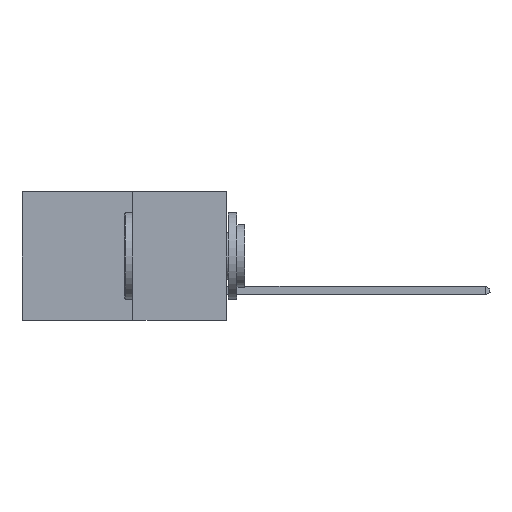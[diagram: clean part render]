
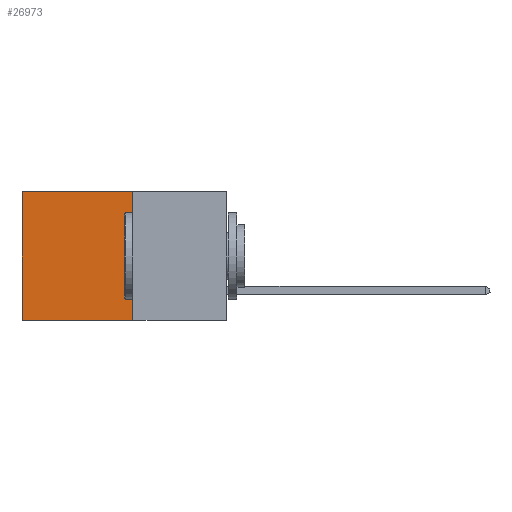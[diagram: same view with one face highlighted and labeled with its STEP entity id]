
A CAD part, left-side view. The second image highlights one B-rep face of the part: STEP entity #26973.
In plain terms, the highlighted planar face has unit normal (-1, 0, 0).
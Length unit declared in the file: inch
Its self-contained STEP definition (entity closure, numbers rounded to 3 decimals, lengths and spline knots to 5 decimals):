
#985 = LINE ( 'NONE', #19650, #26317 ) ;
#1512 = VERTEX_POINT ( 'NONE', #6569 ) ;
#2138 = VECTOR ( 'NONE', #2376, 39.37008 ) ;
#2376 = DIRECTION ( 'NONE',  ( 0., 1., 0. ) ) ;
#3024 = CARTESIAN_POINT ( 'NONE',  ( 0.277, 0.27, -0.37 ) ) ;
#3269 = VERTEX_POINT ( 'NONE', #3748 ) ;
#3719 = DIRECTION ( 'NONE',  ( 0., 1., 0. ) ) ;
#3748 = CARTESIAN_POINT ( 'NONE',  ( 0.277, 0.59, 0. ) ) ;
#5266 = LINE ( 'NONE', #24656, #11060 ) ;
#5448 = DIRECTION ( 'NONE',  ( 0., 0., -1. ) ) ;
#6569 = CARTESIAN_POINT ( 'NONE',  ( 0.277, 0.59, -0.37 ) ) ;
#6896 = LINE ( 'NONE', #23371, #25718 ) ;
#8676 = LINE ( 'NONE', #26833, #2138 ) ;
#9875 = AXIS2_PLACEMENT_3D ( 'NONE', #3024, #20206, #5448 ) ;
#10342 = VERTEX_POINT ( 'NONE', #30927 ) ;
#11060 = VECTOR ( 'NONE', #17388, 39.37008 ) ;
#11911 = EDGE_CURVE ( 'NONE', #22059, #10342, #5266, .T. ) ;
#12427 = ORIENTED_EDGE ( 'NONE', *, *, #29948, .F. ) ;
#14367 = EDGE_CURVE ( 'NONE', #3269, #1512, #985, .T. ) ;
#17032 = ORIENTED_EDGE ( 'NONE', *, *, #27685, .T. ) ;
#17388 = DIRECTION ( 'NONE',  ( 0., 0., -1. ) ) ;
#17759 = PLANE ( 'NONE',  #9875 ) ;
#19650 = CARTESIAN_POINT ( 'NONE',  ( 0.277, 0.59, -0.37 ) ) ;
#20057 = EDGE_LOOP ( 'NONE', ( #22193, #12427, #22409, #17032 ) ) ;
#20206 = DIRECTION ( 'NONE',  ( 1., 0., 0. ) ) ;
#21181 = FACE_OUTER_BOUND ( 'NONE', #20057, .T. ) ;
#22059 = VERTEX_POINT ( 'NONE', #22129 ) ;
#22129 = CARTESIAN_POINT ( 'NONE',  ( 0.277, 0.27, 0. ) ) ;
#22193 = ORIENTED_EDGE ( 'NONE', *, *, #14367, .T. ) ;
#22409 = ORIENTED_EDGE ( 'NONE', *, *, #11911, .F. ) ;
#23371 = CARTESIAN_POINT ( 'NONE',  ( 0.277, 0.27, 0. ) ) ;
#24656 = CARTESIAN_POINT ( 'NONE',  ( 0.277, 0.27, -0.37 ) ) ;
#25718 = VECTOR ( 'NONE', #3719, 39.37008 ) ;
#26317 = VECTOR ( 'NONE', #26999, 39.37008 ) ;
#26833 = CARTESIAN_POINT ( 'NONE',  ( 0.277, 0.27, -0.37 ) ) ;
#26973 = ADVANCED_FACE ( 'NONE', ( #21181 ), #17759, .F. ) ;
#26999 = DIRECTION ( 'NONE',  ( 0., 0., -1. ) ) ;
#27685 = EDGE_CURVE ( 'NONE', #22059, #3269, #6896, .T. ) ;
#29948 = EDGE_CURVE ( 'NONE', #10342, #1512, #8676, .T. ) ;
#30927 = CARTESIAN_POINT ( 'NONE',  ( 0.277, 0.27, -0.37 ) ) ;
